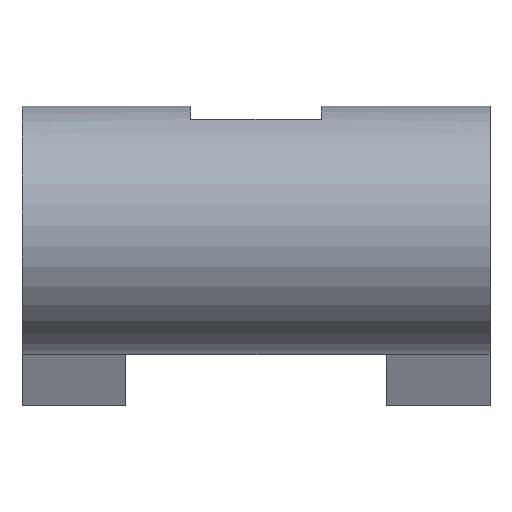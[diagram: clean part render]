
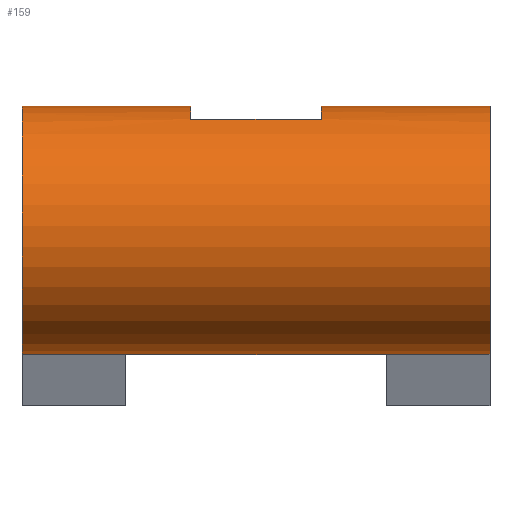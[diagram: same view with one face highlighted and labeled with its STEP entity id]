
A CAD part, front view. The second image highlights one B-rep face of the part: STEP entity #159.
In plain terms, the highlighted cylindrical face has radius 6.053 mm (diameter 12.105 mm), a partial arc.
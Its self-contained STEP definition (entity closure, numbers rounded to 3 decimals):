
#7 = DIRECTION ( 'NONE',  ( 1., 0., 0. ) ) ;
#13 = DIRECTION ( 'NONE',  ( 1., 0., 0. ) ) ;
#21 = VECTOR ( 'NONE', #7, 1000. ) ;
#39 = DIRECTION ( 'NONE',  ( 1., 0., 0. ) ) ;
#52 = LINE ( 'NONE', #172, #649 ) ;
#89 = CARTESIAN_POINT ( 'NONE',  ( 3.175, -38.329, 8.552 ) ) ;
#91 = AXIS2_PLACEMENT_3D ( 'NONE', #89, #629, #168 ) ;
#95 = CIRCLE ( 'NONE', #428, 6.052 ) ;
#97 = DIRECTION ( 'NONE',  ( 1., 0., 0. ) ) ;
#110 = CARTESIAN_POINT ( 'NONE',  ( -6.35, -38.329, 8.552 ) ) ;
#136 = EDGE_CURVE ( 'NONE', #860, #355, #713, .T. ) ;
#143 = EDGE_CURVE ( 'NONE', #699, #918, #95, .T. ) ;
#147 = LINE ( 'NONE', #360, #584 ) ;
#159 = ADVANCED_FACE ( 'NONE', ( #493 ), #261, .T. ) ;
#168 = DIRECTION ( 'NONE',  ( 0., 0., -1. ) ) ;
#172 = CARTESIAN_POINT ( 'NONE',  ( -11.405, -38.329, 14.605 ) ) ;
#198 = DIRECTION ( 'NONE',  ( 0., 0., 1. ) ) ;
#199 = ORIENTED_EDGE ( 'NONE', *, *, #308, .F. ) ;
#203 = EDGE_CURVE ( 'NONE', #973, #862, #640, .T. ) ;
#204 = CARTESIAN_POINT ( 'NONE',  ( -11.405, -38.329, 8.552 ) ) ;
#224 = ORIENTED_EDGE ( 'NONE', *, *, #143, .F. ) ;
#226 = DIRECTION ( 'NONE',  ( 1., 0., 0. ) ) ;
#236 = EDGE_CURVE ( 'NONE', #819, #973, #574, .T. ) ;
#242 = CARTESIAN_POINT ( 'NONE',  ( -3.175, -38.329, 8.552 ) ) ;
#246 = LINE ( 'NONE', #495, #21 ) ;
#261 = CYLINDRICAL_SURFACE ( 'NONE', #627, 6.052 ) ;
#263 = EDGE_CURVE ( 'NONE', #781, #862, #329, .T. ) ;
#270 = ORIENTED_EDGE ( 'NONE', *, *, #673, .T. ) ;
#280 = AXIS2_PLACEMENT_3D ( 'NONE', #110, #661, #198 ) ;
#302 = EDGE_CURVE ( 'NONE', #892, #819, #52, .T. ) ;
#308 = EDGE_CURVE ( 'NONE', #781, #504, #246, .T. ) ;
#321 = CARTESIAN_POINT ( 'NONE',  ( 11.405, -38.791, 2.518 ) ) ;
#325 = CARTESIAN_POINT ( 'NONE',  ( -11.405, -38.329, 8.552 ) ) ;
#329 = CIRCLE ( 'NONE', #91, 6.052 ) ;
#332 = DIRECTION ( 'NONE',  ( 0., 0., -1. ) ) ;
#355 = VERTEX_POINT ( 'NONE', #500 ) ;
#360 = CARTESIAN_POINT ( 'NONE',  ( -33.027, -38.329, 2.5 ) ) ;
#376 = EDGE_CURVE ( 'NONE', #703, #355, #934, .T. ) ;
#378 = DIRECTION ( 'NONE',  ( 1., 0., 0. ) ) ;
#389 = EDGE_CURVE ( 'NONE', #860, #918, #147, .T. ) ;
#404 = DIRECTION ( 'NONE',  ( 0., 0., -1. ) ) ;
#428 = AXIS2_PLACEMENT_3D ( 'NONE', #523, #39, #591 ) ;
#435 = DIRECTION ( 'NONE',  ( 1., 0., 0. ) ) ;
#439 = AXIS2_PLACEMENT_3D ( 'NONE', #690, #226, #760 ) ;
#442 = ORIENTED_EDGE ( 'NONE', *, *, #376, .T. ) ;
#443 = CARTESIAN_POINT ( 'NONE',  ( 6.35, -38.329, 2.5 ) ) ;
#451 = ORIENTED_EDGE ( 'NONE', *, *, #236, .F. ) ;
#483 = ORIENTED_EDGE ( 'NONE', *, *, #389, .T. ) ;
#493 = FACE_OUTER_BOUND ( 'NONE', #839, .T. ) ;
#495 = CARTESIAN_POINT ( 'NONE',  ( -11.405, -38.329, 14.605 ) ) ;
#500 = CARTESIAN_POINT ( 'NONE',  ( -6.35, -38.791, 2.518 ) ) ;
#504 = VERTEX_POINT ( 'NONE', #656 ) ;
#523 = CARTESIAN_POINT ( 'NONE',  ( 6.35, -38.329, 8.552 ) ) ;
#524 = EDGE_CURVE ( 'NONE', #699, #680, #663, .T. ) ;
#555 = CIRCLE ( 'NONE', #439, 6.052 ) ;
#574 = CIRCLE ( 'NONE', #818, 6.052 ) ;
#584 = VECTOR ( 'NONE', #857, 1000. ) ;
#591 = DIRECTION ( 'NONE',  ( 0., 0., 1. ) ) ;
#606 = EDGE_CURVE ( 'NONE', #504, #680, #555, .T. ) ;
#627 = AXIS2_PLACEMENT_3D ( 'NONE', #204, #378, #666 ) ;
#629 = DIRECTION ( 'NONE',  ( 1., 0., 0. ) ) ;
#638 = VECTOR ( 'NONE', #435, 1000. ) ;
#640 = LINE ( 'NONE', #695, #790 ) ;
#649 = VECTOR ( 'NONE', #97, 1000. ) ;
#654 = ORIENTED_EDGE ( 'NONE', *, *, #524, .T. ) ;
#656 = CARTESIAN_POINT ( 'NONE',  ( 11.405, -38.329, 14.605 ) ) ;
#661 = DIRECTION ( 'NONE',  ( -1., 0., 0. ) ) ;
#663 = LINE ( 'NONE', #873, #638 ) ;
#666 = DIRECTION ( 'NONE',  ( 0., 0., -1. ) ) ;
#673 = EDGE_CURVE ( 'NONE', #892, #703, #889, .T. ) ;
#680 = VERTEX_POINT ( 'NONE', #321 ) ;
#690 = CARTESIAN_POINT ( 'NONE',  ( 11.405, -38.329, 8.552 ) ) ;
#694 = AXIS2_PLACEMENT_3D ( 'NONE', #325, #832, #404 ) ;
#695 = CARTESIAN_POINT ( 'NONE',  ( -11.405, -41.027, 13.97 ) ) ;
#696 = CARTESIAN_POINT ( 'NONE',  ( 6.35, -38.791, 2.518 ) ) ;
#699 = VERTEX_POINT ( 'NONE', #696 ) ;
#703 = VERTEX_POINT ( 'NONE', #768 ) ;
#708 = CARTESIAN_POINT ( 'NONE',  ( 3.175, -38.329, 14.605 ) ) ;
#713 = CIRCLE ( 'NONE', #280, 6.052 ) ;
#721 = CARTESIAN_POINT ( 'NONE',  ( -11.405, -38.791, 2.518 ) ) ;
#729 = ORIENTED_EDGE ( 'NONE', *, *, #136, .F. ) ;
#741 = ORIENTED_EDGE ( 'NONE', *, *, #302, .F. ) ;
#747 = ORIENTED_EDGE ( 'NONE', *, *, #263, .T. ) ;
#753 = VECTOR ( 'NONE', #13, 1000. ) ;
#760 = DIRECTION ( 'NONE',  ( 0., 0., -1. ) ) ;
#768 = CARTESIAN_POINT ( 'NONE',  ( -11.405, -38.791, 2.518 ) ) ;
#771 = DIRECTION ( 'NONE',  ( 1., 0., 0. ) ) ;
#774 = ORIENTED_EDGE ( 'NONE', *, *, #606, .F. ) ;
#775 = CARTESIAN_POINT ( 'NONE',  ( -3.175, -38.329, 14.605 ) ) ;
#781 = VERTEX_POINT ( 'NONE', #708 ) ;
#790 = VECTOR ( 'NONE', #830, 1000. ) ;
#793 = ORIENTED_EDGE ( 'NONE', *, *, #203, .F. ) ;
#818 = AXIS2_PLACEMENT_3D ( 'NONE', #242, #771, #332 ) ;
#819 = VERTEX_POINT ( 'NONE', #775 ) ;
#830 = DIRECTION ( 'NONE',  ( 1., 0., 0. ) ) ;
#832 = DIRECTION ( 'NONE',  ( 1., 0., 0. ) ) ;
#839 = EDGE_LOOP ( 'NONE', ( #741, #270, #442, #729, #483, #224, #654, #774, #199, #747, #793, #451 ) ) ;
#843 = CARTESIAN_POINT ( 'NONE',  ( -6.35, -38.329, 2.5 ) ) ;
#857 = DIRECTION ( 'NONE',  ( 1., 0., 0. ) ) ;
#860 = VERTEX_POINT ( 'NONE', #843 ) ;
#862 = VERTEX_POINT ( 'NONE', #912 ) ;
#873 = CARTESIAN_POINT ( 'NONE',  ( -11.405, -38.791, 2.518 ) ) ;
#881 = CARTESIAN_POINT ( 'NONE',  ( -11.405, -38.329, 14.605 ) ) ;
#883 = CARTESIAN_POINT ( 'NONE',  ( -3.175, -41.027, 13.97 ) ) ;
#889 = CIRCLE ( 'NONE', #694, 6.052 ) ;
#892 = VERTEX_POINT ( 'NONE', #881 ) ;
#912 = CARTESIAN_POINT ( 'NONE',  ( 3.175, -41.027, 13.97 ) ) ;
#918 = VERTEX_POINT ( 'NONE', #443 ) ;
#934 = LINE ( 'NONE', #721, #753 ) ;
#973 = VERTEX_POINT ( 'NONE', #883 ) ;
